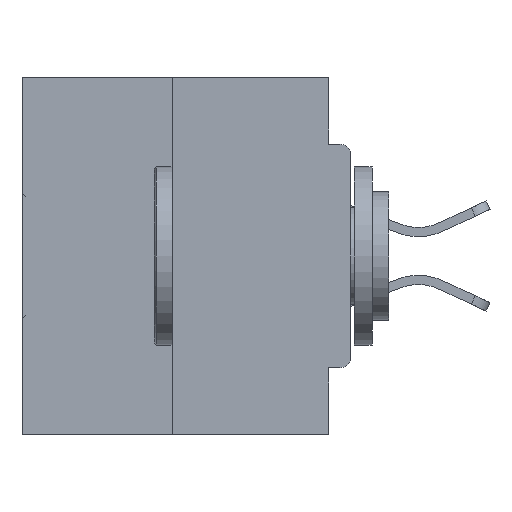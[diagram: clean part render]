
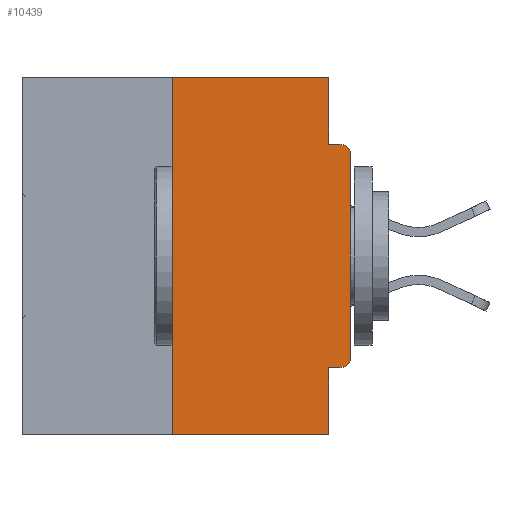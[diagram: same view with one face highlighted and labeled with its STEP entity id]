
A CAD part, left-side view. The second image highlights one B-rep face of the part: STEP entity #10439.
In plain terms, the highlighted planar face has unit normal (-1, 0, 0).
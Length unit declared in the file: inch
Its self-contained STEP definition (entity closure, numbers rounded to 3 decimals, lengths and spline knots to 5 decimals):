
#1196 = LINE ( 'NONE', #35712, #14426 ) ;
#1906 = CARTESIAN_POINT ( 'NONE',  ( 0., 0.015, -0.3915 ) ) ;
#2263 = VERTEX_POINT ( 'NONE', #17985 ) ;
#2527 = VERTEX_POINT ( 'NONE', #43725 ) ;
#2542 = CIRCLE ( 'NONE', #41936, 0.015 ) ;
#2739 = CARTESIAN_POINT ( 'NONE',  ( 0., 0.25, 0. ) ) ;
#2975 = LINE ( 'NONE', #37353, #35857 ) ;
#3727 = DIRECTION ( 'NONE',  ( 0., 0., -1. ) ) ;
#4172 = CARTESIAN_POINT ( 'NONE',  ( 0., 0., 0. ) ) ;
#4478 = CARTESIAN_POINT ( 'NONE',  ( 0., 0.015, -0.0935 ) ) ;
#4594 = VERTEX_POINT ( 'NONE', #15649 ) ;
#4821 = DIRECTION ( 'NONE',  ( 0., 0., -1. ) ) ;
#4882 = DIRECTION ( 'NONE',  ( -1., 0., 0. ) ) ;
#4982 = CARTESIAN_POINT ( 'NONE',  ( 0., 0.25, 0. ) ) ;
#5638 = DIRECTION ( 'NONE',  ( 0., 0., -1. ) ) ;
#6198 = VECTOR ( 'NONE', #4821, 39.37008 ) ;
#6617 = VECTOR ( 'NONE', #9296, 39.37008 ) ;
#7569 = VERTEX_POINT ( 'NONE', #17721 ) ;
#9296 = DIRECTION ( 'NONE',  ( 0., 0., 1. ) ) ;
#10138 = VECTOR ( 'NONE', #41641, 39.37008 ) ;
#10191 = LINE ( 'NONE', #27935, #36631 ) ;
#10439 = ADVANCED_FACE ( 'NONE', ( #34622 ), #36991, .F. ) ;
#12267 = CARTESIAN_POINT ( 'NONE',  ( 0., 0.031, 0. ) ) ;
#14078 = ORIENTED_EDGE ( 'NONE', *, *, #30734, .T. ) ;
#14426 = VECTOR ( 'NONE', #25656, 39.37008 ) ;
#15649 = CARTESIAN_POINT ( 'NONE',  ( 0., 0.031, -0.4065 ) ) ;
#16608 = CARTESIAN_POINT ( 'NONE',  ( 0., 0.031, -0.0935 ) ) ;
#16771 = LINE ( 'NONE', #25417, #6198 ) ;
#16872 = EDGE_CURVE ( 'NONE', #22847, #4594, #36459, .T. ) ;
#16974 = EDGE_CURVE ( 'NONE', #34891, #30224, #2542, .T. ) ;
#17721 = CARTESIAN_POINT ( 'NONE',  ( 0., 0.031, -0.5 ) ) ;
#17985 = CARTESIAN_POINT ( 'NONE',  ( 0., 0.25, -0.5 ) ) ;
#19977 = DIRECTION ( 'NONE',  ( 1., 0., 0. ) ) ;
#20648 = EDGE_CURVE ( 'NONE', #2263, #7569, #1196, .T. ) ;
#21047 = VECTOR ( 'NONE', #5638, 39.37008 ) ;
#21755 = AXIS2_PLACEMENT_3D ( 'NONE', #1906, #4882, #25327 ) ;
#22847 = VERTEX_POINT ( 'NONE', #42895 ) ;
#23231 = DIRECTION ( 'NONE',  ( 0., 0., -1. ) ) ;
#23239 = EDGE_CURVE ( 'NONE', #32177, #32523, #35383, .T. ) ;
#24034 = DIRECTION ( 'NONE',  ( 0., -1., 0. ) ) ;
#25327 = DIRECTION ( 'NONE',  ( 0., 0., -1. ) ) ;
#25417 = CARTESIAN_POINT ( 'NONE',  ( 0., 0.031, -0.5 ) ) ;
#25656 = DIRECTION ( 'NONE',  ( 0., -1., 0. ) ) ;
#27172 = VERTEX_POINT ( 'NONE', #4982 ) ;
#27437 = CIRCLE ( 'NONE', #21755, 0.015 ) ;
#27449 = CARTESIAN_POINT ( 'NONE',  ( 0., 0.015, -0.1085 ) ) ;
#27492 = ORIENTED_EDGE ( 'NONE', *, *, #38842, .F. ) ;
#27505 = CARTESIAN_POINT ( 'NONE',  ( 0., 0., -0.4065 ) ) ;
#27852 = LINE ( 'NONE', #2739, #6617 ) ;
#27935 = CARTESIAN_POINT ( 'NONE',  ( 0., 0.46, 0. ) ) ;
#28671 = EDGE_CURVE ( 'NONE', #2527, #34891, #39263, .T. ) ;
#28977 = ORIENTED_EDGE ( 'NONE', *, *, #16872, .F. ) ;
#30224 = VERTEX_POINT ( 'NONE', #4478 ) ;
#30590 = DIRECTION ( 'NONE',  ( -1., 0., 0. ) ) ;
#30734 = EDGE_CURVE ( 'NONE', #22847, #2527, #27437, .T. ) ;
#31308 = EDGE_CURVE ( 'NONE', #32523, #30224, #2975, .T. ) ;
#31309 = ORIENTED_EDGE ( 'NONE', *, *, #31308, .F. ) ;
#32177 = VERTEX_POINT ( 'NONE', #33419 ) ;
#32523 = VERTEX_POINT ( 'NONE', #16608 ) ;
#32824 = ORIENTED_EDGE ( 'NONE', *, *, #23239, .F. ) ;
#33419 = CARTESIAN_POINT ( 'NONE',  ( 0., 0.031, 0. ) ) ;
#34310 = DIRECTION ( 'NONE',  ( 0., 1., 0. ) ) ;
#34340 = VECTOR ( 'NONE', #34310, 39.37008 ) ;
#34425 = CARTESIAN_POINT ( 'NONE',  ( 0., 0., -0.1085 ) ) ;
#34622 = FACE_OUTER_BOUND ( 'NONE', #43786, .T. ) ;
#34651 = ORIENTED_EDGE ( 'NONE', *, *, #28671, .T. ) ;
#34891 = VERTEX_POINT ( 'NONE', #34425 ) ;
#34916 = EDGE_CURVE ( 'NONE', #27172, #32177, #10191, .T. ) ;
#35383 = LINE ( 'NONE', #12267, #21047 ) ;
#35712 = CARTESIAN_POINT ( 'NONE',  ( 0., 0.46, -0.5 ) ) ;
#35857 = VECTOR ( 'NONE', #24034, 39.37008 ) ;
#36459 = LINE ( 'NONE', #27505, #34340 ) ;
#36631 = VECTOR ( 'NONE', #38095, 39.37008 ) ;
#36991 = PLANE ( 'NONE',  #37527 ) ;
#37353 = CARTESIAN_POINT ( 'NONE',  ( 0., 0., -0.0935 ) ) ;
#37527 = AXIS2_PLACEMENT_3D ( 'NONE', #40660, #19977, #23231 ) ;
#37603 = ORIENTED_EDGE ( 'NONE', *, *, #34916, .F. ) ;
#37939 = ORIENTED_EDGE ( 'NONE', *, *, #20648, .T. ) ;
#38095 = DIRECTION ( 'NONE',  ( 0., -1., 0. ) ) ;
#38842 = EDGE_CURVE ( 'NONE', #2263, #27172, #27852, .T. ) ;
#39263 = LINE ( 'NONE', #4172, #10138 ) ;
#40660 = CARTESIAN_POINT ( 'NONE',  ( 0., 0.46, 0. ) ) ;
#41163 = ORIENTED_EDGE ( 'NONE', *, *, #16974, .T. ) ;
#41569 = EDGE_CURVE ( 'NONE', #4594, #7569, #16771, .T. ) ;
#41641 = DIRECTION ( 'NONE',  ( 0., 0., 1. ) ) ;
#41936 = AXIS2_PLACEMENT_3D ( 'NONE', #27449, #30590, #3727 ) ;
#42598 = ORIENTED_EDGE ( 'NONE', *, *, #41569, .F. ) ;
#42895 = CARTESIAN_POINT ( 'NONE',  ( 0., 0.015, -0.4065 ) ) ;
#43725 = CARTESIAN_POINT ( 'NONE',  ( 0., 0., -0.3915 ) ) ;
#43786 = EDGE_LOOP ( 'NONE', ( #37603, #27492, #37939, #42598, #28977, #14078, #34651, #41163, #31309, #32824 ) ) ;
